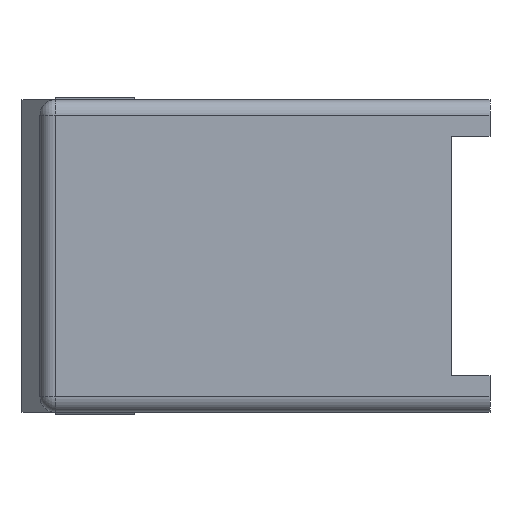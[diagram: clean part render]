
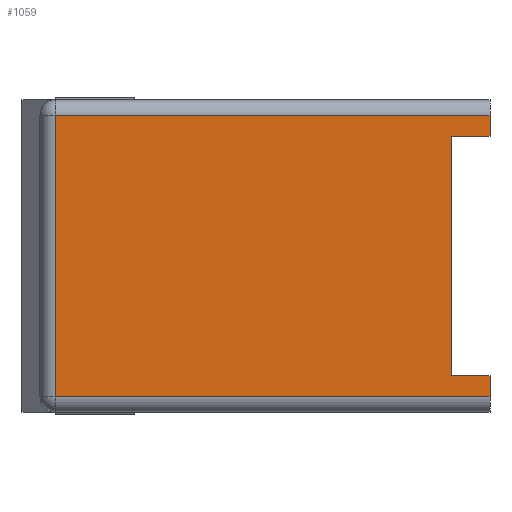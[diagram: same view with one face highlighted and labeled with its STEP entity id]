
A CAD part, left-side view. The second image highlights one B-rep face of the part: STEP entity #1059.
In plain terms, the highlighted planar face has unit normal (-1, 0, 0).
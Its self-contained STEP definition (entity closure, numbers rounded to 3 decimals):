
#37 = EDGE_CURVE ( 'NONE', #859, #1108, #227, .T. ) ;
#42 = CARTESIAN_POINT ( 'NONE',  ( 0., 0., -31.344 ) ) ;
#50 = DIRECTION ( 'NONE',  ( 0., 0., 1. ) ) ;
#53 = EDGE_CURVE ( 'NONE', #1981, #790, #1391, .T. ) ;
#93 = LINE ( 'NONE', #662, #549 ) ;
#182 = DIRECTION ( 'NONE',  ( 0., -1., 0. ) ) ;
#199 = VECTOR ( 'NONE', #1987, 1000. ) ;
#212 = LINE ( 'NONE', #576, #872 ) ;
#223 = VERTEX_POINT ( 'NONE', #1097 ) ;
#227 = LINE ( 'NONE', #2188, #978 ) ;
#243 = CARTESIAN_POINT ( 'NONE',  ( 0., 43.51, -1.575 ) ) ;
#305 = ORIENTED_EDGE ( 'NONE', *, *, #2211, .T. ) ;
#355 = ORIENTED_EDGE ( 'NONE', *, *, #2138, .T. ) ;
#367 = ORIENTED_EDGE ( 'NONE', *, *, #1219, .T. ) ;
#549 = VECTOR ( 'NONE', #50, 1000. ) ;
#576 = CARTESIAN_POINT ( 'NONE',  ( 0., 0., -31.344 ) ) ;
#653 = CARTESIAN_POINT ( 'NONE',  ( 0., 43.51, -31.344 ) ) ;
#662 = CARTESIAN_POINT ( 'NONE',  ( 0., 0., -31.344 ) ) ;
#748 = CARTESIAN_POINT ( 'NONE',  ( 0., 0., -29.769 ) ) ;
#790 = VERTEX_POINT ( 'NONE', #1081 ) ;
#859 = VERTEX_POINT ( 'NONE', #2092 ) ;
#872 = VECTOR ( 'NONE', #996, 1000. ) ;
#920 = ORIENTED_EDGE ( 'NONE', *, *, #37, .F. ) ;
#952 = VECTOR ( 'NONE', #1528, 1000. ) ;
#970 = LINE ( 'NONE', #2309, #1365 ) ;
#978 = VECTOR ( 'NONE', #1795, 1000. ) ;
#996 = DIRECTION ( 'NONE',  ( 0., 0., 1. ) ) ;
#1059 = ADVANCED_FACE ( 'NONE', ( #1796 ), #2190, .T. ) ;
#1081 = CARTESIAN_POINT ( 'NONE',  ( 0., 43.51, -29.769 ) ) ;
#1097 = CARTESIAN_POINT ( 'NONE',  ( 0., 0., -1.575 ) ) ;
#1108 = VERTEX_POINT ( 'NONE', #1440 ) ;
#1118 = DIRECTION ( 'NONE',  ( 0., 0., -1. ) ) ;
#1160 = CARTESIAN_POINT ( 'NONE',  ( 0., 0., -3.683 ) ) ;
#1164 = LINE ( 'NONE', #1756, #952 ) ;
#1188 = DIRECTION ( 'NONE',  ( -1., 0., 0. ) ) ;
#1213 = VERTEX_POINT ( 'NONE', #1722 ) ;
#1214 = ORIENTED_EDGE ( 'NONE', *, *, #1776, .F. ) ;
#1219 = EDGE_CURVE ( 'NONE', #790, #1530, #2147, .T. ) ;
#1271 = CARTESIAN_POINT ( 'NONE',  ( 0., 3.81, -27.661 ) ) ;
#1302 = ORIENTED_EDGE ( 'NONE', *, *, #2359, .T. ) ;
#1327 = AXIS2_PLACEMENT_3D ( 'NONE', #42, #1188, #2200 ) ;
#1365 = VECTOR ( 'NONE', #1567, 1000. ) ;
#1391 = LINE ( 'NONE', #653, #199 ) ;
#1440 = CARTESIAN_POINT ( 'NONE',  ( 0., 0., -27.661 ) ) ;
#1468 = VECTOR ( 'NONE', #1118, 1000. ) ;
#1498 = CARTESIAN_POINT ( 'NONE',  ( 0., 0., -29.769 ) ) ;
#1528 = DIRECTION ( 'NONE',  ( 0., 1., 0. ) ) ;
#1530 = VERTEX_POINT ( 'NONE', #1498 ) ;
#1567 = DIRECTION ( 'NONE',  ( 0., 1., 0. ) ) ;
#1570 = EDGE_CURVE ( 'NONE', #1213, #859, #2081, .T. ) ;
#1636 = EDGE_LOOP ( 'NONE', ( #2389, #367, #355, #920, #2435, #1214, #305, #1302 ) ) ;
#1722 = CARTESIAN_POINT ( 'NONE',  ( 0., 3.81, -3.683 ) ) ;
#1756 = CARTESIAN_POINT ( 'NONE',  ( 0., 3.81, -3.683 ) ) ;
#1776 = EDGE_CURVE ( 'NONE', #2199, #1213, #1164, .T. ) ;
#1795 = DIRECTION ( 'NONE',  ( 0., -1., 0. ) ) ;
#1796 = FACE_OUTER_BOUND ( 'NONE', #1636, .T. ) ;
#1981 = VERTEX_POINT ( 'NONE', #243 ) ;
#1987 = DIRECTION ( 'NONE',  ( 0., 0., -1. ) ) ;
#2081 = LINE ( 'NONE', #1271, #1468 ) ;
#2092 = CARTESIAN_POINT ( 'NONE',  ( 0., 3.81, -27.661 ) ) ;
#2138 = EDGE_CURVE ( 'NONE', #1530, #1108, #212, .T. ) ;
#2147 = LINE ( 'NONE', #748, #2245 ) ;
#2188 = CARTESIAN_POINT ( 'NONE',  ( 0., 3.81, -27.661 ) ) ;
#2190 = PLANE ( 'NONE',  #1327 ) ;
#2199 = VERTEX_POINT ( 'NONE', #1160 ) ;
#2200 = DIRECTION ( 'NONE',  ( 0., 0., 1. ) ) ;
#2211 = EDGE_CURVE ( 'NONE', #2199, #223, #93, .T. ) ;
#2245 = VECTOR ( 'NONE', #182, 1000. ) ;
#2309 = CARTESIAN_POINT ( 'NONE',  ( 0., 45.085, -1.575 ) ) ;
#2359 = EDGE_CURVE ( 'NONE', #223, #1981, #970, .T. ) ;
#2389 = ORIENTED_EDGE ( 'NONE', *, *, #53, .T. ) ;
#2435 = ORIENTED_EDGE ( 'NONE', *, *, #1570, .F. ) ;
